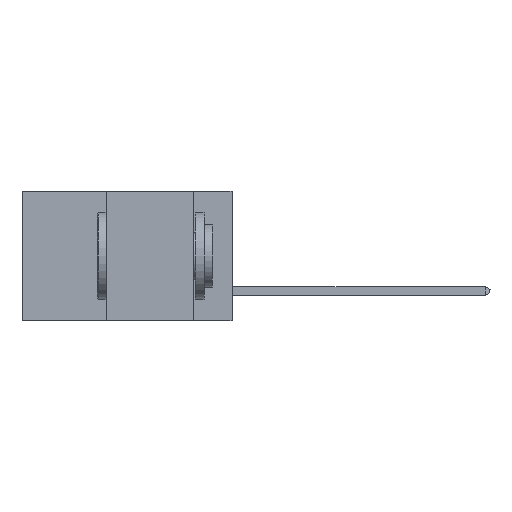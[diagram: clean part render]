
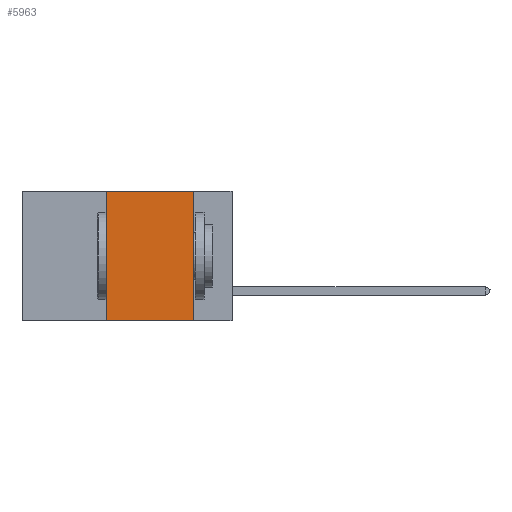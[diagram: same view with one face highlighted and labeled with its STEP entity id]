
A CAD part, left-side view. The second image highlights one B-rep face of the part: STEP entity #5963.
In plain terms, the highlighted planar face has unit normal (-1, 0, 0).
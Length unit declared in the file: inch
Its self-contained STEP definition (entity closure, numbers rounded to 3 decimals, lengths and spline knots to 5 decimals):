
#1661 = VERTEX_POINT ( 'NONE', #27836 ) ;
#3361 = CARTESIAN_POINT ( 'NONE',  ( 0., 0.36, 0. ) ) ;
#4040 = CARTESIAN_POINT ( 'NONE',  ( 0., 0.6, -0.37 ) ) ;
#4471 = CARTESIAN_POINT ( 'NONE',  ( 0., 0.11, 0. ) ) ;
#4591 = DIRECTION ( 'NONE',  ( 0., 0., -1. ) ) ;
#5004 = CARTESIAN_POINT ( 'NONE',  ( 0., 0.11, -0.37 ) ) ;
#5706 = CARTESIAN_POINT ( 'NONE',  ( 0., 0.6, 0. ) ) ;
#5963 = ADVANCED_FACE ( 'NONE', ( #15689 ), #23670, .F. ) ;
#6202 = CARTESIAN_POINT ( 'NONE',  ( 0., 0.11, 0. ) ) ;
#7021 = ORIENTED_EDGE ( 'NONE', *, *, #22720, .F. ) ;
#7710 = EDGE_CURVE ( 'NONE', #1661, #28029, #27531, .T. ) ;
#8227 = DIRECTION ( 'NONE',  ( 0., -1., 0. ) ) ;
#9224 = CARTESIAN_POINT ( 'NONE',  ( 0., 0.36, 0. ) ) ;
#9265 = DIRECTION ( 'NONE',  ( 0., 0., -1. ) ) ;
#9410 = EDGE_CURVE ( 'NONE', #1661, #9906, #9810, .T. ) ;
#9810 = LINE ( 'NONE', #3361, #18797 ) ;
#9906 = VERTEX_POINT ( 'NONE', #9224 ) ;
#10053 = AXIS2_PLACEMENT_3D ( 'NONE', #27969, #13965, #4591 ) ;
#11240 = DIRECTION ( 'NONE',  ( 0., -1., 0. ) ) ;
#13344 = ORIENTED_EDGE ( 'NONE', *, *, #9410, .F. ) ;
#13670 = LINE ( 'NONE', #4471, #26282 ) ;
#13965 = DIRECTION ( 'NONE',  ( 1., 0., 0. ) ) ;
#15689 = FACE_OUTER_BOUND ( 'NONE', #30130, .T. ) ;
#18797 = VECTOR ( 'NONE', #26909, 39.37008 ) ;
#21559 = VERTEX_POINT ( 'NONE', #6202 ) ;
#22562 = VECTOR ( 'NONE', #8227, 39.37008 ) ;
#22720 = EDGE_CURVE ( 'NONE', #21559, #28029, #13670, .T. ) ;
#23670 = PLANE ( 'NONE',  #10053 ) ;
#24798 = LINE ( 'NONE', #5706, #22562 ) ;
#25547 = EDGE_CURVE ( 'NONE', #9906, #21559, #24798, .T. ) ;
#26055 = ORIENTED_EDGE ( 'NONE', *, *, #7710, .T. ) ;
#26282 = VECTOR ( 'NONE', #9265, 39.37008 ) ;
#26909 = DIRECTION ( 'NONE',  ( 0., 0., 1. ) ) ;
#27531 = LINE ( 'NONE', #4040, #27888 ) ;
#27836 = CARTESIAN_POINT ( 'NONE',  ( 0., 0.36, -0.37 ) ) ;
#27888 = VECTOR ( 'NONE', #11240, 39.37008 ) ;
#27969 = CARTESIAN_POINT ( 'NONE',  ( 0., 0.6, 0. ) ) ;
#28029 = VERTEX_POINT ( 'NONE', #5004 ) ;
#28853 = ORIENTED_EDGE ( 'NONE', *, *, #25547, .F. ) ;
#30130 = EDGE_LOOP ( 'NONE', ( #7021, #28853, #13344, #26055 ) ) ;
